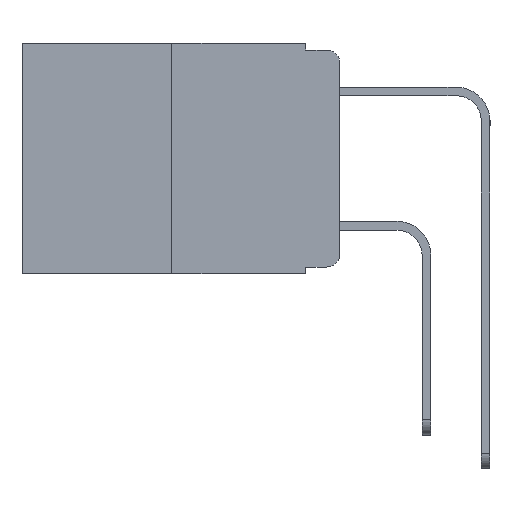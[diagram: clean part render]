
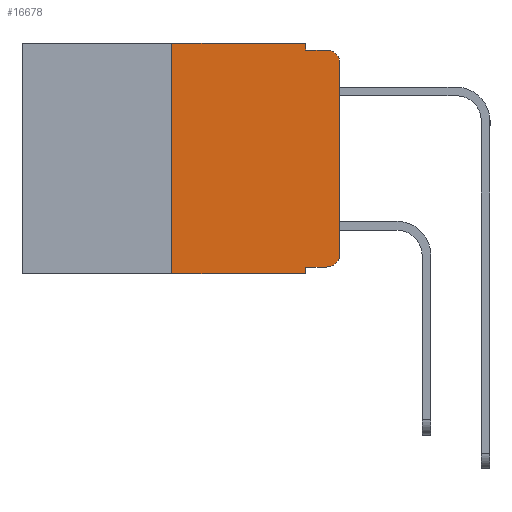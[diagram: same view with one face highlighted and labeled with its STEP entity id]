
A CAD part, left-side view. The second image highlights one B-rep face of the part: STEP entity #16678.
In plain terms, the highlighted planar face has unit normal (-1, 0, 0).
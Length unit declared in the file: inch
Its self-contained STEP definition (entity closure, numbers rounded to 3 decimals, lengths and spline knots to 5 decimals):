
#203 = DIRECTION ( 'NONE',  ( 0., 0., 1. ) ) ;
#557 = EDGE_CURVE ( 'NONE', #12134, #14223, #9806, .T. ) ;
#833 = ORIENTED_EDGE ( 'NONE', *, *, #13116, .T. ) ;
#871 = DIRECTION ( 'NONE',  ( -1., 0., 0. ) ) ;
#1293 = CARTESIAN_POINT ( 'NONE',  ( 0., 0.02, -0.03 ) ) ;
#1344 = DIRECTION ( 'NONE',  ( 0., -1., 0. ) ) ;
#1450 = LINE ( 'NONE', #13774, #7649 ) ;
#1855 = VERTEX_POINT ( 'NONE', #6329 ) ;
#2009 = FACE_OUTER_BOUND ( 'NONE', #16518, .T. ) ;
#2292 = VERTEX_POINT ( 'NONE', #5381 ) ;
#2634 = ORIENTED_EDGE ( 'NONE', *, *, #5106, .F. ) ;
#2680 = DIRECTION ( 'NONE',  ( 0., 0., -1. ) ) ;
#2685 = DIRECTION ( 'NONE',  ( 0., 0., -1. ) ) ;
#2882 = VECTOR ( 'NONE', #203, 39.37008 ) ;
#3308 = CARTESIAN_POINT ( 'NONE',  ( 0., 0., -0.03 ) ) ;
#3375 = LINE ( 'NONE', #10513, #16099 ) ;
#3392 = VERTEX_POINT ( 'NONE', #3308 ) ;
#3412 = ORIENTED_EDGE ( 'NONE', *, *, #557, .F. ) ;
#3554 = VECTOR ( 'NONE', #11725, 39.37008 ) ;
#3814 = CARTESIAN_POINT ( 'NONE',  ( 0., 0.25, 0. ) ) ;
#4232 = EDGE_CURVE ( 'NONE', #4710, #14981, #7288, .T. ) ;
#4261 = VECTOR ( 'NONE', #2685, 39.37008 ) ;
#4274 = ORIENTED_EDGE ( 'NONE', *, *, #16411, .F. ) ;
#4710 = VERTEX_POINT ( 'NONE', #15985 ) ;
#4899 = ORIENTED_EDGE ( 'NONE', *, *, #13918, .F. ) ;
#4945 = VECTOR ( 'NONE', #6792, 39.37008 ) ;
#5106 = EDGE_CURVE ( 'NONE', #14981, #1855, #1450, .T. ) ;
#5284 = VECTOR ( 'NONE', #7646, 39.37008 ) ;
#5381 = CARTESIAN_POINT ( 'NONE',  ( 0., 0.051, -0.343 ) ) ;
#5453 = DIRECTION ( 'NONE',  ( 0., -1., 0. ) ) ;
#6004 = DIRECTION ( 'NONE',  ( 0., -1., 0. ) ) ;
#6329 = CARTESIAN_POINT ( 'NONE',  ( 0., 0.02, -0.01 ) ) ;
#6517 = AXIS2_PLACEMENT_3D ( 'NONE', #10995, #15980, #8481 ) ;
#6537 = VERTEX_POINT ( 'NONE', #15721 ) ;
#6707 = ORIENTED_EDGE ( 'NONE', *, *, #7687, .T. ) ;
#6792 = DIRECTION ( 'NONE',  ( 0., -1., 0. ) ) ;
#7068 = AXIS2_PLACEMENT_3D ( 'NONE', #1293, #10470, #2680 ) ;
#7186 = PLANE ( 'NONE',  #6517 ) ;
#7288 = LINE ( 'NONE', #11917, #4261 ) ;
#7646 = DIRECTION ( 'NONE',  ( 0., 0., 1. ) ) ;
#7649 = VECTOR ( 'NONE', #6004, 39.37008 ) ;
#7687 = EDGE_CURVE ( 'NONE', #3392, #1855, #8611, .T. ) ;
#8203 = CARTESIAN_POINT ( 'NONE',  ( 0., 0.051, -0.333 ) ) ;
#8481 = DIRECTION ( 'NONE',  ( 0., 0., -1. ) ) ;
#8566 = EDGE_CURVE ( 'NONE', #6537, #3392, #15374, .T. ) ;
#8611 = CIRCLE ( 'NONE', #7068, 0.02 ) ;
#8795 = CARTESIAN_POINT ( 'NONE',  ( 0., 0.02, -0.313 ) ) ;
#9143 = ORIENTED_EDGE ( 'NONE', *, *, #13934, .T. ) ;
#9610 = AXIS2_PLACEMENT_3D ( 'NONE', #8795, #871, #10085 ) ;
#9806 = LINE ( 'NONE', #3814, #2882 ) ;
#10085 = DIRECTION ( 'NONE',  ( 0., 0., -1. ) ) ;
#10296 = ORIENTED_EDGE ( 'NONE', *, *, #10495, .T. ) ;
#10450 = CARTESIAN_POINT ( 'NONE',  ( 0., 0.051, 0. ) ) ;
#10470 = DIRECTION ( 'NONE',  ( -1., 0., 0. ) ) ;
#10495 = EDGE_CURVE ( 'NONE', #12134, #2292, #3375, .T. ) ;
#10513 = CARTESIAN_POINT ( 'NONE',  ( 0., 0.473, -0.343 ) ) ;
#10829 = LINE ( 'NONE', #10450, #3554 ) ;
#10995 = CARTESIAN_POINT ( 'NONE',  ( 0., 0.473, 0. ) ) ;
#11557 = CIRCLE ( 'NONE', #9610, 0.02 ) ;
#11725 = DIRECTION ( 'NONE',  ( 0., 0., -1. ) ) ;
#11917 = CARTESIAN_POINT ( 'NONE',  ( 0., 0.051, 0. ) ) ;
#11968 = ORIENTED_EDGE ( 'NONE', *, *, #4232, .F. ) ;
#12134 = VERTEX_POINT ( 'NONE', #14376 ) ;
#12704 = LINE ( 'NONE', #13144, #4945 ) ;
#13016 = VERTEX_POINT ( 'NONE', #16069 ) ;
#13116 = EDGE_CURVE ( 'NONE', #13016, #6537, #11557, .T. ) ;
#13144 = CARTESIAN_POINT ( 'NONE',  ( 0., 0.051, -0.333 ) ) ;
#13478 = LINE ( 'NONE', #15567, #15977 ) ;
#13774 = CARTESIAN_POINT ( 'NONE',  ( 0., 0.051, -0.01 ) ) ;
#13918 = EDGE_CURVE ( 'NONE', #14223, #4710, #13478, .T. ) ;
#13934 = EDGE_CURVE ( 'NONE', #14018, #13016, #12704, .T. ) ;
#13949 = CARTESIAN_POINT ( 'NONE',  ( 0., 0., 0. ) ) ;
#14018 = VERTEX_POINT ( 'NONE', #8203 ) ;
#14223 = VERTEX_POINT ( 'NONE', #15784 ) ;
#14336 = ORIENTED_EDGE ( 'NONE', *, *, #8566, .T. ) ;
#14376 = CARTESIAN_POINT ( 'NONE',  ( 0., 0.25, -0.343 ) ) ;
#14981 = VERTEX_POINT ( 'NONE', #16355 ) ;
#15374 = LINE ( 'NONE', #13949, #5284 ) ;
#15567 = CARTESIAN_POINT ( 'NONE',  ( 0., 0.473, 0. ) ) ;
#15721 = CARTESIAN_POINT ( 'NONE',  ( 0., 0., -0.313 ) ) ;
#15784 = CARTESIAN_POINT ( 'NONE',  ( 0., 0.25, 0. ) ) ;
#15977 = VECTOR ( 'NONE', #5453, 39.37008 ) ;
#15980 = DIRECTION ( 'NONE',  ( 1., 0., 0. ) ) ;
#15985 = CARTESIAN_POINT ( 'NONE',  ( 0., 0.051, 0. ) ) ;
#16069 = CARTESIAN_POINT ( 'NONE',  ( 0., 0.02, -0.333 ) ) ;
#16099 = VECTOR ( 'NONE', #1344, 39.37008 ) ;
#16355 = CARTESIAN_POINT ( 'NONE',  ( 0., 0.051, -0.01 ) ) ;
#16411 = EDGE_CURVE ( 'NONE', #14018, #2292, #10829, .T. ) ;
#16518 = EDGE_LOOP ( 'NONE', ( #14336, #6707, #2634, #11968, #4899, #3412, #10296, #4274, #9143, #833 ) ) ;
#16678 = ADVANCED_FACE ( 'NONE', ( #2009 ), #7186, .F. ) ;
